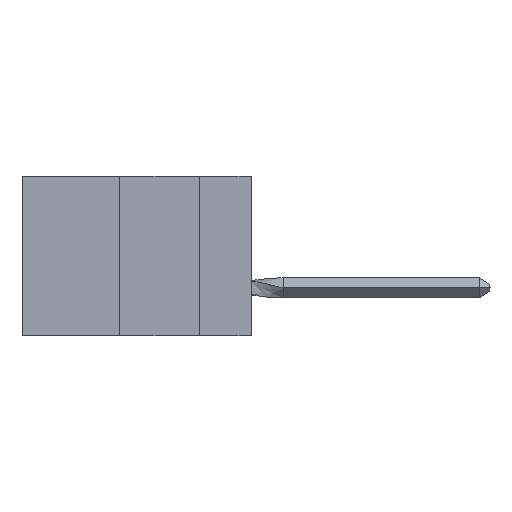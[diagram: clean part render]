
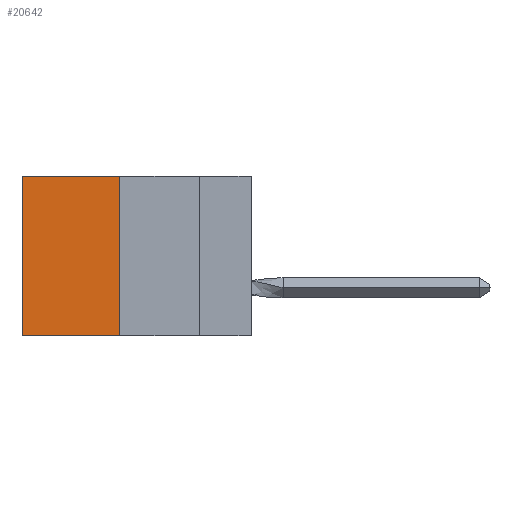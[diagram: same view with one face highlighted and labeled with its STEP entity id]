
A CAD part, left-side view. The second image highlights one B-rep face of the part: STEP entity #20642.
In plain terms, the highlighted planar face has unit normal (-1, 0, 0).
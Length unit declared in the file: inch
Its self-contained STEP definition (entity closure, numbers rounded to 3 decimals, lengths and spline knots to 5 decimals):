
#37 = VECTOR ( 'NONE', #24623, 39.37008 ) ;
#309 = CARTESIAN_POINT ( 'NONE',  ( 0.305, 0.72, -0.5 ) ) ;
#760 = DIRECTION ( 'NONE',  ( 1., 0., 0. ) ) ;
#843 = VECTOR ( 'NONE', #26583, 39.37008 ) ;
#1332 = CARTESIAN_POINT ( 'NONE',  ( 0.305, 0.72, 0. ) ) ;
#2701 = CARTESIAN_POINT ( 'NONE',  ( 0.305, 0.413, -0.5 ) ) ;
#2894 = CARTESIAN_POINT ( 'NONE',  ( 0.305, 0.413, -0.5 ) ) ;
#4482 = CARTESIAN_POINT ( 'NONE',  ( 0.305, 0.413, 0. ) ) ;
#4485 = DIRECTION ( 'NONE',  ( 0., 0., -1. ) ) ;
#5210 = VERTEX_POINT ( 'NONE', #7987 ) ;
#5438 = ORIENTED_EDGE ( 'NONE', *, *, #10251, .F. ) ;
#7200 = LINE ( 'NONE', #29085, #28947 ) ;
#7712 = CARTESIAN_POINT ( 'NONE',  ( 0.305, 0.413, -0.5 ) ) ;
#7987 = CARTESIAN_POINT ( 'NONE',  ( 0.305, 0.413, -0.5 ) ) ;
#8164 = LINE ( 'NONE', #2894, #18003 ) ;
#8794 = LINE ( 'NONE', #4482, #37 ) ;
#9210 = VERTEX_POINT ( 'NONE', #309 ) ;
#9492 = DIRECTION ( 'NONE',  ( 0., 0., -1. ) ) ;
#10132 = DIRECTION ( 'NONE',  ( 0., 0., -1. ) ) ;
#10251 = EDGE_CURVE ( 'NONE', #5210, #9210, #23298, .T. ) ;
#10399 = EDGE_CURVE ( 'NONE', #23701, #5210, #8164, .T. ) ;
#11740 = EDGE_CURVE ( 'NONE', #23701, #24850, #8794, .T. ) ;
#12288 = ORIENTED_EDGE ( 'NONE', *, *, #22948, .T. ) ;
#14387 = CARTESIAN_POINT ( 'NONE',  ( 0.305, 0.413, 0. ) ) ;
#17354 = AXIS2_PLACEMENT_3D ( 'NONE', #7712, #760, #10132 ) ;
#18003 = VECTOR ( 'NONE', #9492, 39.37008 ) ;
#18288 = EDGE_LOOP ( 'NONE', ( #12288, #5438, #27604, #18513 ) ) ;
#18513 = ORIENTED_EDGE ( 'NONE', *, *, #11740, .T. ) ;
#20642 = ADVANCED_FACE ( 'NONE', ( #27672 ), #25736, .F. ) ;
#22948 = EDGE_CURVE ( 'NONE', #24850, #9210, #7200, .T. ) ;
#23298 = LINE ( 'NONE', #2701, #843 ) ;
#23701 = VERTEX_POINT ( 'NONE', #14387 ) ;
#24623 = DIRECTION ( 'NONE',  ( 0., 1., 0. ) ) ;
#24850 = VERTEX_POINT ( 'NONE', #1332 ) ;
#25736 = PLANE ( 'NONE',  #17354 ) ;
#26583 = DIRECTION ( 'NONE',  ( 0., 1., 0. ) ) ;
#27604 = ORIENTED_EDGE ( 'NONE', *, *, #10399, .F. ) ;
#27672 = FACE_OUTER_BOUND ( 'NONE', #18288, .T. ) ;
#28947 = VECTOR ( 'NONE', #4485, 39.37008 ) ;
#29085 = CARTESIAN_POINT ( 'NONE',  ( 0.305, 0.72, -0.5 ) ) ;
